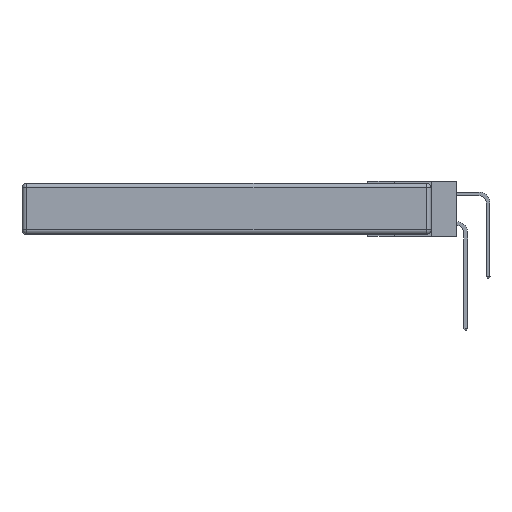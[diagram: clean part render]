
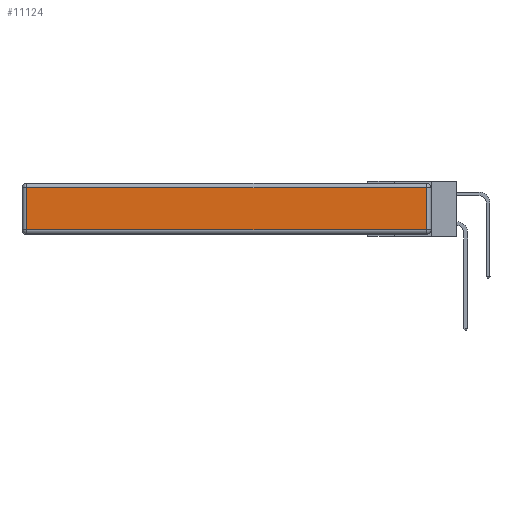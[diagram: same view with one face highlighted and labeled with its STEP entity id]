
A CAD part, left-side view. The second image highlights one B-rep face of the part: STEP entity #11124.
In plain terms, the highlighted planar face has unit normal (-1, 0, 0).
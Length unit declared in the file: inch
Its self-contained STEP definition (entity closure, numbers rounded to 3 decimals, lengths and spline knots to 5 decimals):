
#99 = AXIS2_PLACEMENT_3D ( 'NONE', #3072, #11323, #4245 ) ;
#186 = DIRECTION ( 'NONE',  ( 0., -1., 0. ) ) ;
#885 = VECTOR ( 'NONE', #1298, 39.37008 ) ;
#971 = VERTEX_POINT ( 'NONE', #5612 ) ;
#1017 = CARTESIAN_POINT ( 'NONE',  ( 0., 2.75, -0.03 ) ) ;
#1298 = DIRECTION ( 'NONE',  ( 0., 0., 1. ) ) ;
#1510 = CARTESIAN_POINT ( 'NONE',  ( 0., 2.72, -0.343 ) ) ;
#2037 = VECTOR ( 'NONE', #186, 39.37008 ) ;
#3072 = CARTESIAN_POINT ( 'NONE',  ( 0., 0., -0.343 ) ) ;
#3550 = VERTEX_POINT ( 'NONE', #13864 ) ;
#3650 = CARTESIAN_POINT ( 'NONE',  ( 0., 0.03, -0.343 ) ) ;
#3651 = EDGE_CURVE ( 'NONE', #12235, #5456, #11597, .T. ) ;
#4108 = ORIENTED_EDGE ( 'NONE', *, *, #3651, .T. ) ;
#4245 = DIRECTION ( 'NONE',  ( 0., 0., 1. ) ) ;
#5456 = VERTEX_POINT ( 'NONE', #8259 ) ;
#5612 = CARTESIAN_POINT ( 'NONE',  ( 0., 2.72, -0.03 ) ) ;
#5818 = DIRECTION ( 'NONE',  ( 0., 1., 0. ) ) ;
#6091 = CARTESIAN_POINT ( 'NONE',  ( 0., 0., -0.313 ) ) ;
#6254 = DIRECTION ( 'NONE',  ( 0., 0., -1. ) ) ;
#6343 = LINE ( 'NONE', #1510, #10563 ) ;
#8120 = ORIENTED_EDGE ( 'NONE', *, *, #9452, .T. ) ;
#8259 = CARTESIAN_POINT ( 'NONE',  ( 0., 0.03, -0.03 ) ) ;
#8728 = VECTOR ( 'NONE', #5818, 39.37008 ) ;
#9324 = EDGE_CURVE ( 'NONE', #971, #3550, #6343, .T. ) ;
#9452 = EDGE_CURVE ( 'NONE', #5456, #971, #14248, .T. ) ;
#9821 = CARTESIAN_POINT ( 'NONE',  ( 0., 0.03, -0.313 ) ) ;
#9971 = EDGE_CURVE ( 'NONE', #3550, #12235, #13874, .T. ) ;
#10157 = PLANE ( 'NONE',  #99 ) ;
#10417 = ORIENTED_EDGE ( 'NONE', *, *, #9324, .T. ) ;
#10563 = VECTOR ( 'NONE', #6254, 39.37008 ) ;
#11124 = ADVANCED_FACE ( 'NONE', ( #13092 ), #10157, .T. ) ;
#11323 = DIRECTION ( 'NONE',  ( -1., 0., 0. ) ) ;
#11597 = LINE ( 'NONE', #3650, #885 ) ;
#11626 = EDGE_LOOP ( 'NONE', ( #13548, #4108, #8120, #10417 ) ) ;
#12235 = VERTEX_POINT ( 'NONE', #9821 ) ;
#13092 = FACE_OUTER_BOUND ( 'NONE', #11626, .T. ) ;
#13548 = ORIENTED_EDGE ( 'NONE', *, *, #9971, .T. ) ;
#13864 = CARTESIAN_POINT ( 'NONE',  ( 0., 2.72, -0.313 ) ) ;
#13874 = LINE ( 'NONE', #6091, #2037 ) ;
#14248 = LINE ( 'NONE', #1017, #8728 ) ;
